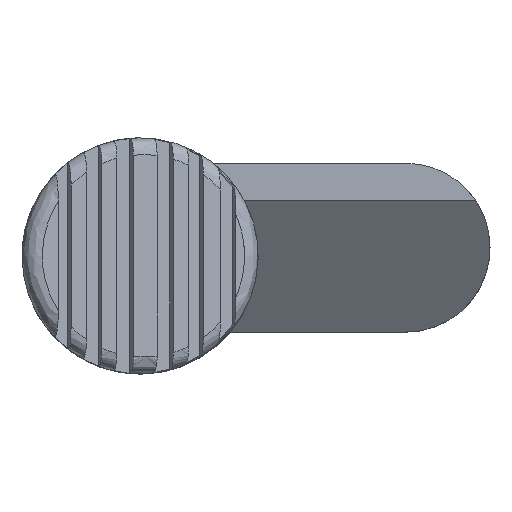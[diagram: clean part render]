
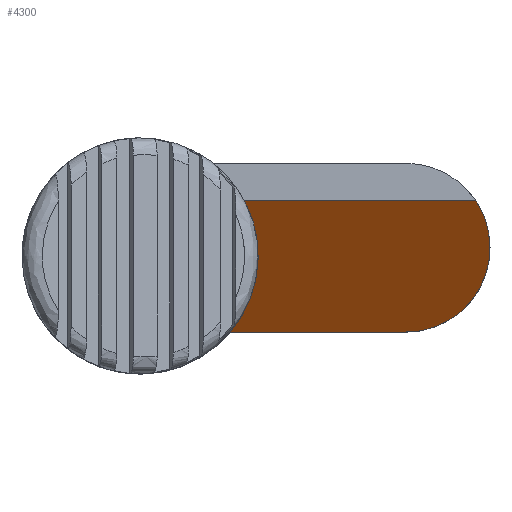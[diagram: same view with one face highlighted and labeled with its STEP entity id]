
A CAD part, top view. The second image highlights one B-rep face of the part: STEP entity #4300.
In plain terms, the highlighted planar face has unit normal (0, -0.595, 0.804).
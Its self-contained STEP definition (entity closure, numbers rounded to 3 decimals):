
#38=ELLIPSE('',#4565,3.11,2.5);
#39=ELLIPSE('',#4566,3.11,2.5);
#42=ELLIPSE('',#4589,3.11,2.5);
#198=FACE_OUTER_BOUND('',#439,.T.);
#439=EDGE_LOOP('',(#2968,#2969,#2970,#2971,#2972));
#813=LINE('',#6469,#1266);
#817=LINE('',#6482,#1270);
#1266=VECTOR('',#5102,8.);
#1270=VECTOR('',#5118,8.);
#1727=VERTEX_POINT('',#6428);
#1728=VERTEX_POINT('',#6430);
#1729=VERTEX_POINT('',#6433);
#1734=VERTEX_POINT('',#6467);
#1737=VERTEX_POINT('',#6474);
#2184=EDGE_CURVE('',#1727,#1728,#38,.T.);
#2186=EDGE_CURVE('',#1728,#1729,#39,.T.);
#2203=EDGE_CURVE('',#1727,#1734,#813,.T.);
#2206=EDGE_CURVE('',#1734,#1737,#42,.T.);
#2210=EDGE_CURVE('',#1737,#1729,#817,.T.);
#2968=ORIENTED_EDGE('',*,*,#2206,.T.);
#2969=ORIENTED_EDGE('',*,*,#2210,.T.);
#2970=ORIENTED_EDGE('',*,*,#2186,.F.);
#2971=ORIENTED_EDGE('',*,*,#2184,.F.);
#2972=ORIENTED_EDGE('',*,*,#2203,.T.);
#4077=PLANE('',#4592);
#4300=ADVANCED_FACE('',(#198),#4077,.T.);
#4565=AXIS2_PLACEMENT_3D('',#6431,#5051,#5052);
#4566=AXIS2_PLACEMENT_3D('',#6434,#5054,#5055);
#4589=AXIS2_PLACEMENT_3D('',#6476,#5108,#5109);
#4592=AXIS2_PLACEMENT_3D('',#6481,#5116,#5117);
#5051=DIRECTION('center_axis',(0.,-0.595,0.804));
#5052=DIRECTION('ref_axis',(0.,-0.804,-0.595));
#5054=DIRECTION('center_axis',(0.,-0.595,0.804));
#5055=DIRECTION('ref_axis',(0.,-0.804,-0.595));
#5102=DIRECTION('',(1.,0.,0.));
#5108=DIRECTION('center_axis',(0.,-0.595,0.804));
#5109=DIRECTION('ref_axis',(0.,-0.804,-0.595));
#5116=DIRECTION('center_axis',(0.,-0.595,0.804));
#5117=DIRECTION('ref_axis',(1.,0.,0.));
#5118=DIRECTION('',(-1.,0.,0.));
#6428=CARTESIAN_POINT('',(0.,-2.5,2.3));
#6430=CARTESIAN_POINT('',(2.5,0.,4.15));
#6431=CARTESIAN_POINT('Origin',(0.,0.,4.15));
#6433=CARTESIAN_POINT('',(2.082,1.384,5.174));
#6434=CARTESIAN_POINT('Origin',(0.,0.,4.15));
#6467=CARTESIAN_POINT('',(8.,-2.5,2.3));
#6469=CARTESIAN_POINT('',(0.,-2.5,2.3));
#6474=CARTESIAN_POINT('',(10.082,1.384,5.174));
#6476=CARTESIAN_POINT('Origin',(8.,0.,4.15));
#6481=CARTESIAN_POINT('Origin',(0.,0.49,4.513));
#6482=CARTESIAN_POINT('',(10.082,1.384,5.174));
